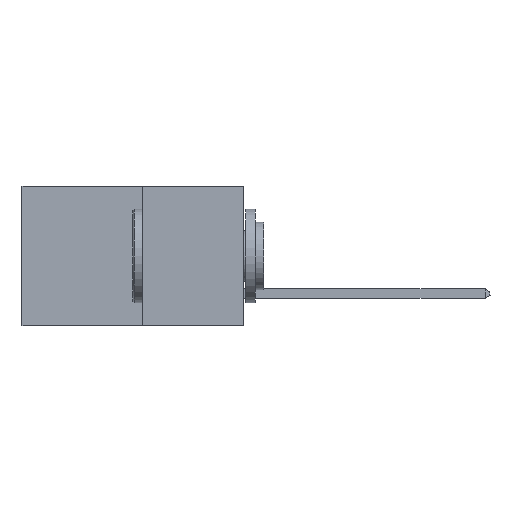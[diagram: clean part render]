
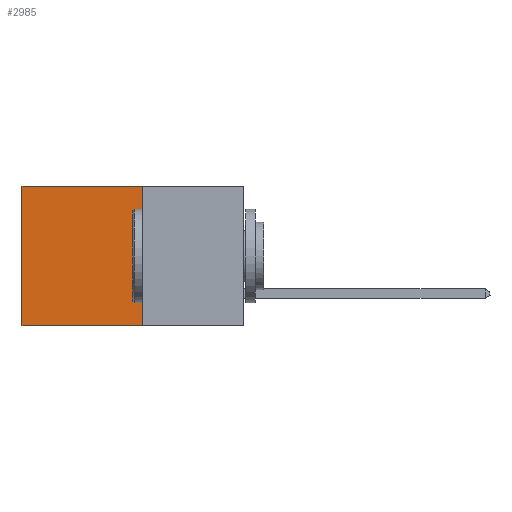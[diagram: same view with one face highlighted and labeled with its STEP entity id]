
A CAD part, left-side view. The second image highlights one B-rep face of the part: STEP entity #2985.
In plain terms, the highlighted planar face has unit normal (-1, 0, 0).
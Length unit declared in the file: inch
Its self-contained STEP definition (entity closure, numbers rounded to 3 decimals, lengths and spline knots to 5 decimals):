
#286 = LINE ( 'NONE', #11669, #5664 ) ;
#1241 = VERTEX_POINT ( 'NONE', #12318 ) ;
#1534 = DIRECTION ( 'NONE',  ( 0., 0., -1. ) ) ;
#1615 = VERTEX_POINT ( 'NONE', #12964 ) ;
#2089 = ORIENTED_EDGE ( 'NONE', *, *, #2967, .T. ) ;
#2777 = FACE_OUTER_BOUND ( 'NONE', #12197, .T. ) ;
#2784 = CARTESIAN_POINT ( 'NONE',  ( 0.277, 0.59, 0. ) ) ;
#2967 = EDGE_CURVE ( 'NONE', #3401, #10894, #286, .T. ) ;
#2985 = ADVANCED_FACE ( 'NONE', ( #2777 ), #10678, .F. ) ;
#3401 = VERTEX_POINT ( 'NONE', #13245 ) ;
#3661 = EDGE_CURVE ( 'NONE', #3401, #1615, #11114, .T. ) ;
#3670 = ORIENTED_EDGE ( 'NONE', *, *, #11997, .T. ) ;
#3703 = CARTESIAN_POINT ( 'NONE',  ( 0.277, 0.59, -0.37 ) ) ;
#3808 = AXIS2_PLACEMENT_3D ( 'NONE', #10570, #10526, #10380 ) ;
#3956 = VECTOR ( 'NONE', #7260, 39.37008 ) ;
#4023 = EDGE_CURVE ( 'NONE', #1615, #1241, #12379, .T. ) ;
#5664 = VECTOR ( 'NONE', #12099, 39.37008 ) ;
#7260 = DIRECTION ( 'NONE',  ( 0., 1., 0. ) ) ;
#7307 = CARTESIAN_POINT ( 'NONE',  ( 0.277, 0.27, -0.37 ) ) ;
#7535 = VECTOR ( 'NONE', #1534, 39.37008 ) ;
#8335 = VECTOR ( 'NONE', #10837, 39.37008 ) ;
#10303 = ORIENTED_EDGE ( 'NONE', *, *, #3661, .F. ) ;
#10380 = DIRECTION ( 'NONE',  ( 0., 0., -1. ) ) ;
#10526 = DIRECTION ( 'NONE',  ( 1., 0., 0. ) ) ;
#10570 = CARTESIAN_POINT ( 'NONE',  ( 0.277, 0.27, -0.37 ) ) ;
#10678 = PLANE ( 'NONE',  #3808 ) ;
#10837 = DIRECTION ( 'NONE',  ( 0., 0., -1. ) ) ;
#10894 = VERTEX_POINT ( 'NONE', #2784 ) ;
#10903 = CARTESIAN_POINT ( 'NONE',  ( 0.277, 0.27, -0.37 ) ) ;
#11114 = LINE ( 'NONE', #10903, #8335 ) ;
#11669 = CARTESIAN_POINT ( 'NONE',  ( 0.277, 0.27, 0. ) ) ;
#11997 = EDGE_CURVE ( 'NONE', #10894, #1241, #13362, .T. ) ;
#12091 = ORIENTED_EDGE ( 'NONE', *, *, #4023, .F. ) ;
#12099 = DIRECTION ( 'NONE',  ( 0., 1., 0. ) ) ;
#12197 = EDGE_LOOP ( 'NONE', ( #3670, #12091, #10303, #2089 ) ) ;
#12318 = CARTESIAN_POINT ( 'NONE',  ( 0.277, 0.59, -0.37 ) ) ;
#12379 = LINE ( 'NONE', #7307, #3956 ) ;
#12964 = CARTESIAN_POINT ( 'NONE',  ( 0.277, 0.27, -0.37 ) ) ;
#13245 = CARTESIAN_POINT ( 'NONE',  ( 0.277, 0.27, 0. ) ) ;
#13362 = LINE ( 'NONE', #3703, #7535 ) ;
